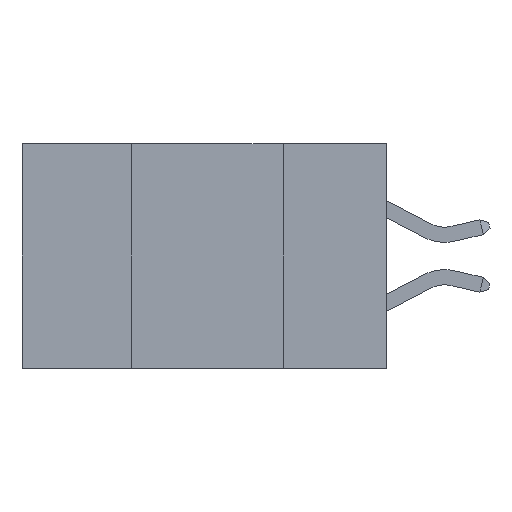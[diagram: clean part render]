
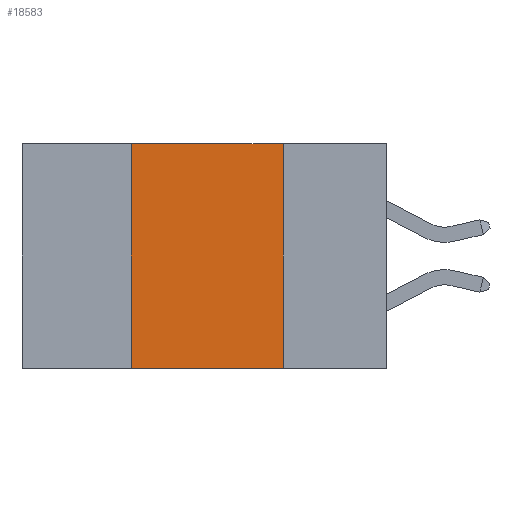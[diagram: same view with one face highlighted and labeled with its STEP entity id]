
A CAD part, left-side view. The second image highlights one B-rep face of the part: STEP entity #18583.
In plain terms, the highlighted planar face has unit normal (-1, 0, 0).
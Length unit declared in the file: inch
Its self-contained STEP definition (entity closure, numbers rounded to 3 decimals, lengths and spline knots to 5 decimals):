
#1354 = PLANE ( 'NONE',  #19520 ) ;
#1386 = LINE ( 'NONE', #21761, #12090 ) ;
#1827 = CARTESIAN_POINT ( 'NONE',  ( 0., 0.17, 0. ) ) ;
#2851 = VERTEX_POINT ( 'NONE', #24279 ) ;
#3073 = ORIENTED_EDGE ( 'NONE', *, *, #20046, .F. ) ;
#3225 = VECTOR ( 'NONE', #3872, 39.37008 ) ;
#3412 = DIRECTION ( 'NONE',  ( 1., 0., 0. ) ) ;
#3872 = DIRECTION ( 'NONE',  ( 0., 0., -1. ) ) ;
#7027 = CARTESIAN_POINT ( 'NONE',  ( 0., 0.6, 0. ) ) ;
#7348 = VERTEX_POINT ( 'NONE', #24426 ) ;
#7395 = LINE ( 'NONE', #7027, #22038 ) ;
#7938 = DIRECTION ( 'NONE',  ( 0., 0., 1. ) ) ;
#8664 = EDGE_CURVE ( 'NONE', #2851, #24358, #1386, .T. ) ;
#8942 = CARTESIAN_POINT ( 'NONE',  ( 0., 0.17, -0.37 ) ) ;
#9846 = DIRECTION ( 'NONE',  ( 0., -1., 0. ) ) ;
#11350 = EDGE_CURVE ( 'NONE', #2851, #13224, #24367, .T. ) ;
#11754 = ORIENTED_EDGE ( 'NONE', *, *, #21667, .F. ) ;
#11827 = ORIENTED_EDGE ( 'NONE', *, *, #11350, .F. ) ;
#12090 = VECTOR ( 'NONE', #9846, 39.37008 ) ;
#13224 = VERTEX_POINT ( 'NONE', #23842 ) ;
#14483 = VECTOR ( 'NONE', #7938, 39.37008 ) ;
#17434 = DIRECTION ( 'NONE',  ( 0., 0., -1. ) ) ;
#17920 = CARTESIAN_POINT ( 'NONE',  ( 0., 0.42, 0. ) ) ;
#18583 = ADVANCED_FACE ( 'NONE', ( #25200 ), #1354, .F. ) ;
#19228 = LINE ( 'NONE', #1827, #3225 ) ;
#19520 = AXIS2_PLACEMENT_3D ( 'NONE', #25183, #3412, #17434 ) ;
#20046 = EDGE_CURVE ( 'NONE', #13224, #7348, #7395, .T. ) ;
#21667 = EDGE_CURVE ( 'NONE', #7348, #24358, #19228, .T. ) ;
#21761 = CARTESIAN_POINT ( 'NONE',  ( 0., 0.6, -0.37 ) ) ;
#22038 = VECTOR ( 'NONE', #22966, 39.37008 ) ;
#22151 = ORIENTED_EDGE ( 'NONE', *, *, #8664, .T. ) ;
#22966 = DIRECTION ( 'NONE',  ( 0., -1., 0. ) ) ;
#23842 = CARTESIAN_POINT ( 'NONE',  ( 0., 0.42, 0. ) ) ;
#24279 = CARTESIAN_POINT ( 'NONE',  ( 0., 0.42, -0.37 ) ) ;
#24358 = VERTEX_POINT ( 'NONE', #8942 ) ;
#24367 = LINE ( 'NONE', #17920, #14483 ) ;
#24426 = CARTESIAN_POINT ( 'NONE',  ( 0., 0.17, 0. ) ) ;
#25183 = CARTESIAN_POINT ( 'NONE',  ( 0., 0.6, 0. ) ) ;
#25200 = FACE_OUTER_BOUND ( 'NONE', #25334, .T. ) ;
#25334 = EDGE_LOOP ( 'NONE', ( #11754, #3073, #11827, #22151 ) ) ;
